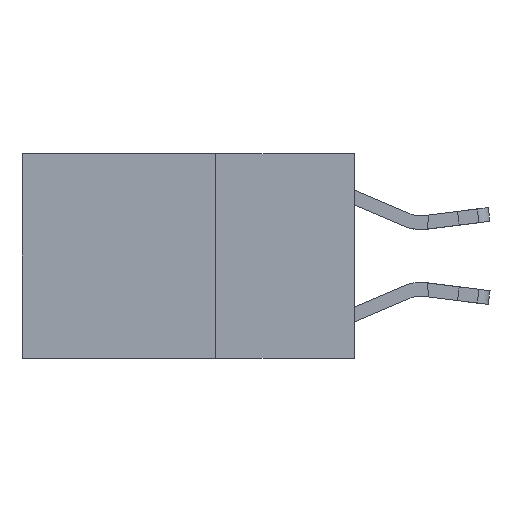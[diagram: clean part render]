
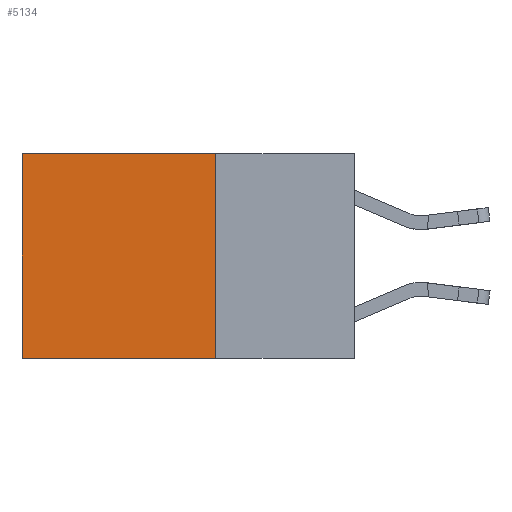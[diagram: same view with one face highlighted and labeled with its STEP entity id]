
A CAD part, left-side view. The second image highlights one B-rep face of the part: STEP entity #5134.
In plain terms, the highlighted planar face has unit normal (-1, 0, 0).
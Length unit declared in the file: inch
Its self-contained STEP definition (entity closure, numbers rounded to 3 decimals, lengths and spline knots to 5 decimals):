
#796 = VECTOR ( 'NONE', #10235, 39.37008 ) ;
#1101 = EDGE_CURVE ( 'NONE', #4793, #2550, #3232, .T. ) ;
#1330 = DIRECTION ( 'NONE',  ( 0., 0., -1. ) ) ;
#1494 = DIRECTION ( 'NONE',  ( 0., 0., -1. ) ) ;
#1782 = CARTESIAN_POINT ( 'NONE',  ( 0.2625, 0.25, 0. ) ) ;
#2550 = VERTEX_POINT ( 'NONE', #17951 ) ;
#3232 = LINE ( 'NONE', #1782, #11647 ) ;
#4793 = VERTEX_POINT ( 'NONE', #17863 ) ;
#4988 = LINE ( 'NONE', #9416, #17362 ) ;
#5134 = ADVANCED_FACE ( 'NONE', ( #16397 ), #17293, .F. ) ;
#5480 = EDGE_CURVE ( 'NONE', #4793, #17675, #4988, .T. ) ;
#5786 = EDGE_CURVE ( 'NONE', #17675, #14452, #15625, .T. ) ;
#5826 = LINE ( 'NONE', #8686, #796 ) ;
#5934 = ORIENTED_EDGE ( 'NONE', *, *, #5786, .F. ) ;
#6459 = CARTESIAN_POINT ( 'NONE',  ( 0.2625, 0.25, 0. ) ) ;
#8686 = CARTESIAN_POINT ( 'NONE',  ( 0.2625, 0.6, 0. ) ) ;
#9155 = CARTESIAN_POINT ( 'NONE',  ( 0.2625, 0.6, -0.37 ) ) ;
#9416 = CARTESIAN_POINT ( 'NONE',  ( 0.2625, 0.25, 0. ) ) ;
#9752 = EDGE_LOOP ( 'NONE', ( #17814, #5934, #10051, #10533 ) ) ;
#10051 = ORIENTED_EDGE ( 'NONE', *, *, #5480, .F. ) ;
#10235 = DIRECTION ( 'NONE',  ( 0., 0., -1. ) ) ;
#10533 = ORIENTED_EDGE ( 'NONE', *, *, #1101, .T. ) ;
#11156 = DIRECTION ( 'NONE',  ( 1., 0., 0. ) ) ;
#11545 = VECTOR ( 'NONE', #11669, 39.37008 ) ;
#11647 = VECTOR ( 'NONE', #14502, 39.37008 ) ;
#11669 = DIRECTION ( 'NONE',  ( 0., 1., 0. ) ) ;
#13103 = AXIS2_PLACEMENT_3D ( 'NONE', #6459, #11156, #1494 ) ;
#14452 = VERTEX_POINT ( 'NONE', #9155 ) ;
#14502 = DIRECTION ( 'NONE',  ( 0., 1., 0. ) ) ;
#15625 = LINE ( 'NONE', #19357, #11545 ) ;
#15864 = EDGE_CURVE ( 'NONE', #2550, #14452, #5826, .T. ) ;
#15920 = CARTESIAN_POINT ( 'NONE',  ( 0.2625, 0.25, -0.37 ) ) ;
#16397 = FACE_OUTER_BOUND ( 'NONE', #9752, .T. ) ;
#17293 = PLANE ( 'NONE',  #13103 ) ;
#17362 = VECTOR ( 'NONE', #1330, 39.37008 ) ;
#17675 = VERTEX_POINT ( 'NONE', #15920 ) ;
#17814 = ORIENTED_EDGE ( 'NONE', *, *, #15864, .T. ) ;
#17863 = CARTESIAN_POINT ( 'NONE',  ( 0.2625, 0.25, 0. ) ) ;
#17951 = CARTESIAN_POINT ( 'NONE',  ( 0.2625, 0.6, 0. ) ) ;
#19357 = CARTESIAN_POINT ( 'NONE',  ( 0.2625, 0.25, -0.37 ) ) ;
